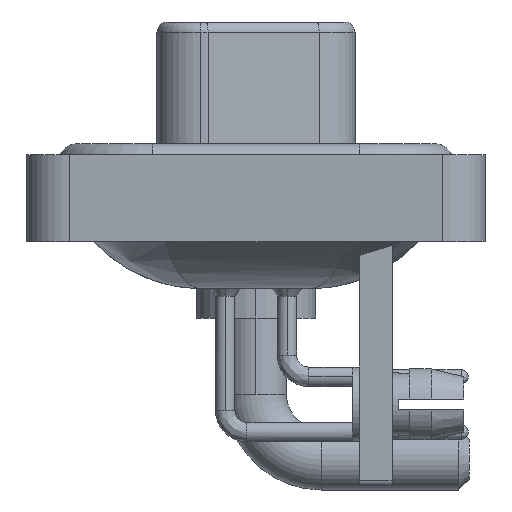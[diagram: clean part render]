
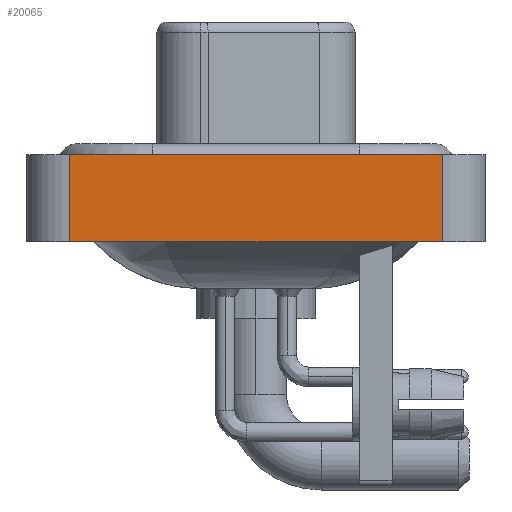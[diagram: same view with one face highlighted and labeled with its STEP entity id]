
A CAD part, left-side view. The second image highlights one B-rep face of the part: STEP entity #20065.
In plain terms, the highlighted planar face has unit normal (-1, 0, 0).
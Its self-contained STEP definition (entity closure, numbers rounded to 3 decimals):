
#402 = ORIENTED_EDGE ( 'NONE', *, *, #7427, .F. ) ;
#464 = DIRECTION ( 'NONE',  ( 0., -1., 0. ) ) ;
#1020 = CARTESIAN_POINT ( 'NONE',  ( -7.3, 8.55, -3.6 ) ) ;
#1597 = CARTESIAN_POINT ( 'NONE',  ( -7.3, -8.55, -3.6 ) ) ;
#1819 = CARTESIAN_POINT ( 'NONE',  ( -7.3, 8.55, 0.4 ) ) ;
#2820 = VECTOR ( 'NONE', #21162, 1000. ) ;
#3525 = VERTEX_POINT ( 'NONE', #1819 ) ;
#4085 = EDGE_LOOP ( 'NONE', ( #9194, #9936, #402, #21562 ) ) ;
#4331 = LINE ( 'NONE', #16988, #2820 ) ;
#4984 = LINE ( 'NONE', #13647, #24159 ) ;
#5831 = EDGE_CURVE ( 'NONE', #16519, #13960, #19842, .T. ) ;
#7151 = DIRECTION ( 'NONE',  ( -1., 0., 0. ) ) ;
#7427 = EDGE_CURVE ( 'NONE', #16519, #3525, #18437, .T. ) ;
#7753 = VERTEX_POINT ( 'NONE', #24960 ) ;
#9194 = ORIENTED_EDGE ( 'NONE', *, *, #16173, .T. ) ;
#9936 = ORIENTED_EDGE ( 'NONE', *, *, #20031, .F. ) ;
#11461 = CARTESIAN_POINT ( 'NONE',  ( -7.3, -8.55, -3.6 ) ) ;
#13647 = CARTESIAN_POINT ( 'NONE',  ( -7.3, -8.55, 0.4 ) ) ;
#13960 = VERTEX_POINT ( 'NONE', #1597 ) ;
#14072 = AXIS2_PLACEMENT_3D ( 'NONE', #11461, #7151, #26825 ) ;
#15796 = FACE_OUTER_BOUND ( 'NONE', #4085, .T. ) ;
#15892 = VECTOR ( 'NONE', #464, 1000. ) ;
#16173 = EDGE_CURVE ( 'NONE', #13960, #7753, #4331, .T. ) ;
#16519 = VERTEX_POINT ( 'NONE', #1020 ) ;
#16988 = CARTESIAN_POINT ( 'NONE',  ( -7.3, -8.55, -3.6 ) ) ;
#17593 = VECTOR ( 'NONE', #27032, 1000. ) ;
#18312 = CARTESIAN_POINT ( 'NONE',  ( -7.3, 8.55, -3.6 ) ) ;
#18437 = LINE ( 'NONE', #18312, #17593 ) ;
#19842 = LINE ( 'NONE', #22309, #15892 ) ;
#19961 = DIRECTION ( 'NONE',  ( 0., -1., 0. ) ) ;
#20031 = EDGE_CURVE ( 'NONE', #3525, #7753, #4984, .T. ) ;
#20065 = ADVANCED_FACE ( 'NONE', ( #15796 ), #24542, .T. ) ;
#21162 = DIRECTION ( 'NONE',  ( 0., 0., 1. ) ) ;
#21562 = ORIENTED_EDGE ( 'NONE', *, *, #5831, .T. ) ;
#22309 = CARTESIAN_POINT ( 'NONE',  ( -7.3, -8.55, -3.6 ) ) ;
#24159 = VECTOR ( 'NONE', #19961, 1000. ) ;
#24542 = PLANE ( 'NONE',  #14072 ) ;
#24960 = CARTESIAN_POINT ( 'NONE',  ( -7.3, -8.55, 0.4 ) ) ;
#26825 = DIRECTION ( 'NONE',  ( 0., 0., 1. ) ) ;
#27032 = DIRECTION ( 'NONE',  ( 0., 0., 1. ) ) ;
